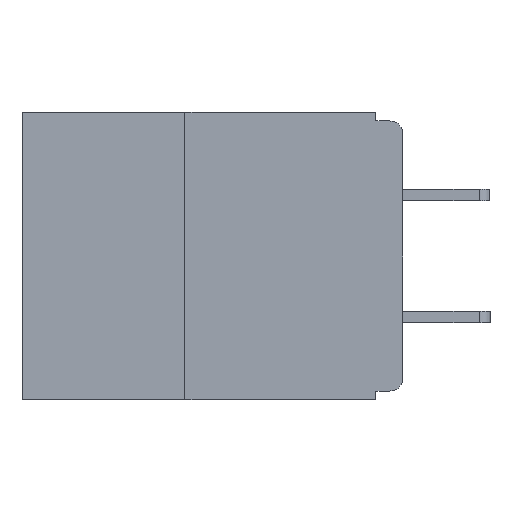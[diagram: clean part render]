
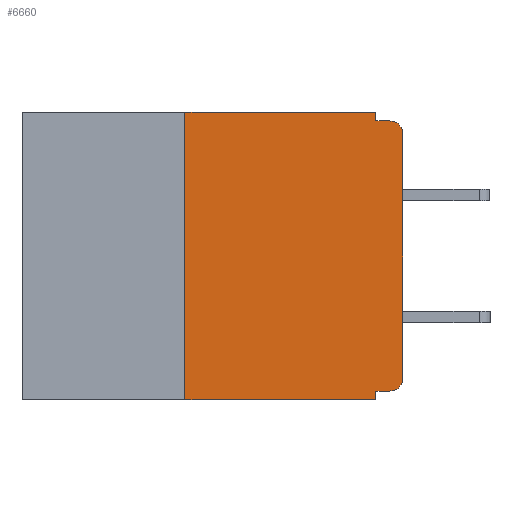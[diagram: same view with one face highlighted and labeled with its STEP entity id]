
A CAD part, left-side view. The second image highlights one B-rep face of the part: STEP entity #6660.
In plain terms, the highlighted planar face has unit normal (-1, 0, 0).
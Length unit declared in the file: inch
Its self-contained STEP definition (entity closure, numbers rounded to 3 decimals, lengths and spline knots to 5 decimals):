
#93 = ORIENTED_EDGE ( 'NONE', *, *, #11425, .F. ) ;
#107 = VERTEX_POINT ( 'NONE', #8745 ) ;
#460 = LINE ( 'NONE', #6826, #1142 ) ;
#498 = VERTEX_POINT ( 'NONE', #13001 ) ;
#636 = EDGE_LOOP ( 'NONE', ( #10490, #2718, #5725, #11526, #93, #12198, #3769, #9675, #1139, #7479 ) ) ;
#819 = VECTOR ( 'NONE', #7079, 39.37008 ) ;
#1139 = ORIENTED_EDGE ( 'NONE', *, *, #8184, .F. ) ;
#1142 = VECTOR ( 'NONE', #2677, 39.37008 ) ;
#1223 = EDGE_CURVE ( 'NONE', #5165, #107, #9629, .T. ) ;
#2677 = DIRECTION ( 'NONE',  ( 0., -1., 0. ) ) ;
#2698 = AXIS2_PLACEMENT_3D ( 'NONE', #9019, #10344, #13897 ) ;
#2718 = ORIENTED_EDGE ( 'NONE', *, *, #8066, .T. ) ;
#3137 = AXIS2_PLACEMENT_3D ( 'NONE', #13719, #13563, #13538 ) ;
#3139 = VERTEX_POINT ( 'NONE', #8970 ) ;
#3310 = EDGE_CURVE ( 'NONE', #12706, #6674, #3788, .T. ) ;
#3706 = FACE_OUTER_BOUND ( 'NONE', #636, .T. ) ;
#3769 = ORIENTED_EDGE ( 'NONE', *, *, #3310, .T. ) ;
#3788 = LINE ( 'NONE', #11513, #12548 ) ;
#3798 = EDGE_CURVE ( 'NONE', #498, #5744, #460, .T. ) ;
#4035 = CARTESIAN_POINT ( 'NONE',  ( 0., 0.031, 0. ) ) ;
#4330 = VERTEX_POINT ( 'NONE', #10485 ) ;
#4585 = LINE ( 'NONE', #12140, #7227 ) ;
#5014 = CARTESIAN_POINT ( 'NONE',  ( 0., 0.015, -0.305 ) ) ;
#5165 = VERTEX_POINT ( 'NONE', #6563 ) ;
#5296 = VECTOR ( 'NONE', #12768, 39.37008 ) ;
#5725 = ORIENTED_EDGE ( 'NONE', *, *, #3798, .F. ) ;
#5744 = VERTEX_POINT ( 'NONE', #7208 ) ;
#6148 = DIRECTION ( 'NONE',  ( 0., 0., -1. ) ) ;
#6345 = DIRECTION ( 'NONE',  ( 0., 0., 1. ) ) ;
#6368 = VECTOR ( 'NONE', #6345, 39.37008 ) ;
#6527 = CARTESIAN_POINT ( 'NONE',  ( 0., 0.437, 0. ) ) ;
#6563 = CARTESIAN_POINT ( 'NONE',  ( 0., 0., -0.305 ) ) ;
#6648 = LINE ( 'NONE', #4035, #9237 ) ;
#6660 = ADVANCED_FACE ( 'NONE', ( #3706 ), #13684, .F. ) ;
#6674 = VERTEX_POINT ( 'NONE', #13401 ) ;
#6765 = EDGE_CURVE ( 'NONE', #12213, #6674, #13954, .T. ) ;
#6785 = LINE ( 'NONE', #7034, #819 ) ;
#6826 = CARTESIAN_POINT ( 'NONE',  ( 0., 0., -0.01 ) ) ;
#6836 = EDGE_CURVE ( 'NONE', #12706, #12927, #4585, .T. ) ;
#7034 = CARTESIAN_POINT ( 'NONE',  ( 0., 0., -0.32 ) ) ;
#7079 = DIRECTION ( 'NONE',  ( 0., 1., 0. ) ) ;
#7208 = CARTESIAN_POINT ( 'NONE',  ( 0., 0.015, -0.01 ) ) ;
#7227 = VECTOR ( 'NONE', #12157, 39.37008 ) ;
#7345 = DIRECTION ( 'NONE',  ( 0., -1., 0. ) ) ;
#7479 = ORIENTED_EDGE ( 'NONE', *, *, #13142, .T. ) ;
#7572 = LINE ( 'NONE', #6527, #12615 ) ;
#8066 = EDGE_CURVE ( 'NONE', #107, #5744, #11044, .T. ) ;
#8184 = EDGE_CURVE ( 'NONE', #4330, #12213, #6785, .T. ) ;
#8251 = AXIS2_PLACEMENT_3D ( 'NONE', #5014, #12659, #6148 ) ;
#8745 = CARTESIAN_POINT ( 'NONE',  ( 0., 0., -0.025 ) ) ;
#8970 = CARTESIAN_POINT ( 'NONE',  ( 0., 0.031, 0. ) ) ;
#9019 = CARTESIAN_POINT ( 'NONE',  ( 0., 0.015, -0.025 ) ) ;
#9237 = VECTOR ( 'NONE', #13845, 39.37008 ) ;
#9629 = LINE ( 'NONE', #10741, #6368 ) ;
#9675 = ORIENTED_EDGE ( 'NONE', *, *, #6765, .F. ) ;
#10046 = CARTESIAN_POINT ( 'NONE',  ( 0., 0.25, 0. ) ) ;
#10344 = DIRECTION ( 'NONE',  ( -1., 0., 0. ) ) ;
#10485 = CARTESIAN_POINT ( 'NONE',  ( 0., 0.015, -0.32 ) ) ;
#10490 = ORIENTED_EDGE ( 'NONE', *, *, #1223, .T. ) ;
#10741 = CARTESIAN_POINT ( 'NONE',  ( 0., 0., 0. ) ) ;
#10832 = CARTESIAN_POINT ( 'NONE',  ( 0., 0.031, -0.32 ) ) ;
#11044 = CIRCLE ( 'NONE', #2698, 0.015 ) ;
#11425 = EDGE_CURVE ( 'NONE', #12927, #3139, #7572, .T. ) ;
#11513 = CARTESIAN_POINT ( 'NONE',  ( 0., 0.437, -0.33 ) ) ;
#11526 = ORIENTED_EDGE ( 'NONE', *, *, #13243, .F. ) ;
#12140 = CARTESIAN_POINT ( 'NONE',  ( 0., 0.25, -0.33 ) ) ;
#12157 = DIRECTION ( 'NONE',  ( 0., 0., 1. ) ) ;
#12198 = ORIENTED_EDGE ( 'NONE', *, *, #6836, .F. ) ;
#12213 = VERTEX_POINT ( 'NONE', #10832 ) ;
#12548 = VECTOR ( 'NONE', #7345, 39.37008 ) ;
#12615 = VECTOR ( 'NONE', #13017, 39.37008 ) ;
#12659 = DIRECTION ( 'NONE',  ( -1., 0., 0. ) ) ;
#12706 = VERTEX_POINT ( 'NONE', #12913 ) ;
#12764 = CARTESIAN_POINT ( 'NONE',  ( 0., 0.031, -0.33 ) ) ;
#12768 = DIRECTION ( 'NONE',  ( 0., 0., -1. ) ) ;
#12913 = CARTESIAN_POINT ( 'NONE',  ( 0., 0.25, -0.33 ) ) ;
#12927 = VERTEX_POINT ( 'NONE', #10046 ) ;
#13001 = CARTESIAN_POINT ( 'NONE',  ( 0., 0.031, -0.01 ) ) ;
#13017 = DIRECTION ( 'NONE',  ( 0., -1., 0. ) ) ;
#13142 = EDGE_CURVE ( 'NONE', #4330, #5165, #13418, .T. ) ;
#13243 = EDGE_CURVE ( 'NONE', #3139, #498, #6648, .T. ) ;
#13401 = CARTESIAN_POINT ( 'NONE',  ( 0., 0.031, -0.33 ) ) ;
#13418 = CIRCLE ( 'NONE', #8251, 0.015 ) ;
#13538 = DIRECTION ( 'NONE',  ( 0., 0., -1. ) ) ;
#13563 = DIRECTION ( 'NONE',  ( 1., 0., 0. ) ) ;
#13684 = PLANE ( 'NONE',  #3137 ) ;
#13719 = CARTESIAN_POINT ( 'NONE',  ( 0., 0.437, 0. ) ) ;
#13845 = DIRECTION ( 'NONE',  ( 0., 0., -1. ) ) ;
#13897 = DIRECTION ( 'NONE',  ( 0., 0., -1. ) ) ;
#13954 = LINE ( 'NONE', #12764, #5296 ) ;
